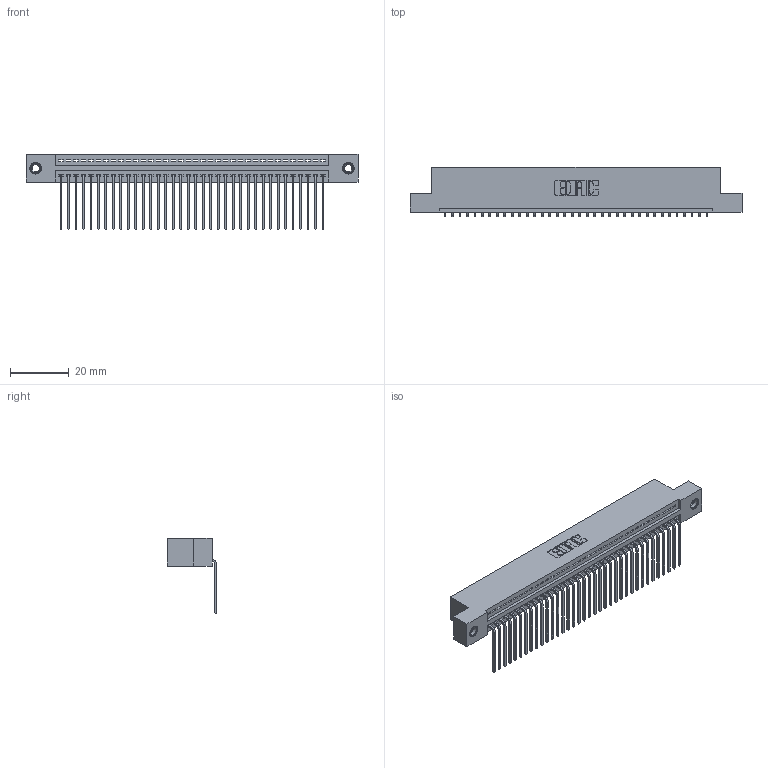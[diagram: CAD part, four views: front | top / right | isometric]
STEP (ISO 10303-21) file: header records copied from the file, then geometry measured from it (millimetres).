
FILE_DESCRIPTION (( 'STEP AP203' ), '1' );
FILE_NAME ('395-036-559-107.STEP', '2018-11-13T21:42:38', ( '' ), ( '' ), 'SwSTEP 2.0', 'SolidWorks 2016', '' );
FILE_SCHEMA (( 'CONFIG_CONTROL_DESIGN' ));
Length unit declared in the file: inch
Products named in the file (4): 395-036-559-107; 345-250-001_345-250-005-103; 345 Part_Flush Mounting Lugs - 0.156 Dia-TI; 345-292-001_558 559 Tail - 1
Assembly tree (39 placements, depth 2):
  395-036-559-107
    345 Part_Flush Mounting Lugs - 0.156 Dia-TI
    345-292-001_558 559 Tail - 1  x36
    345-250-001_345-250-005-103  x2
Bounding box: 112.65 x 16.75 x 25.53 mm (x, y, z)
Volume: 10756.8 mm3; surface area: 14950.6 mm2
Topology: 39 solids, 39 shells, 2346 faces, 7029 edges, 4630 vertices
Faces by surface type: plane 1624, cylinder 706, cone 12, torus 4
Entity records: 29172 total; most frequent: CARTESIAN_POINT 5035, ORIENTED_EDGE 4998, DIRECTION 4433, EDGE_CURVE 2499, VECTOR 2203, LINE 2203, VERTEX_POINT 1660, AXIS2_PLACEMENT_3D 1115
